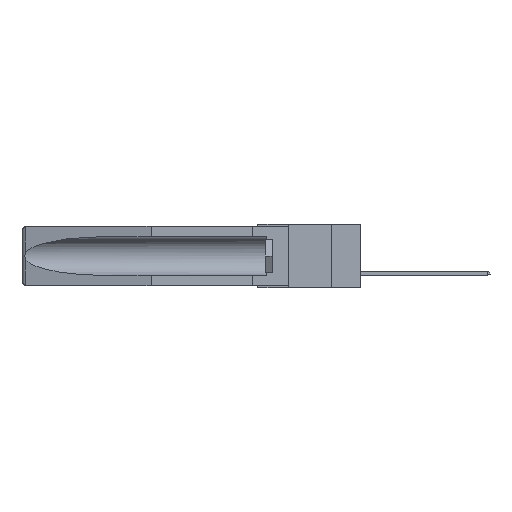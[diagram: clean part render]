
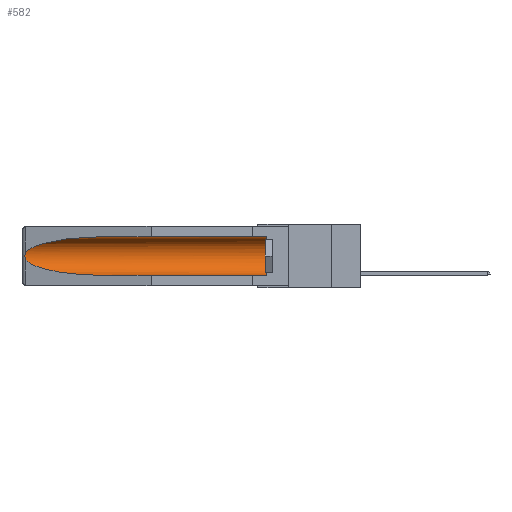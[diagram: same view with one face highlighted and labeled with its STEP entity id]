
A CAD part, left-side view. The second image highlights one B-rep face of the part: STEP entity #582.
In plain terms, the highlighted cylindrical face has radius 2.857 mm (diameter 5.715 mm), a partial arc.
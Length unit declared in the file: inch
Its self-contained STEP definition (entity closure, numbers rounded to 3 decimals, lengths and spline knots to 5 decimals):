
#582 = ADVANCED_FACE ( 'NONE', ( #4923 ), #21378, .F. ) ;
#949 = VECTOR ( 'NONE', #17998, 39.37008 ) ;
#1473 = DIRECTION ( 'NONE',  ( 0., -1., 0. ) ) ;
#1710 = VERTEX_POINT ( 'NONE', #6869 ) ;
#1951 = CARTESIAN_POINT ( 'NONE',  ( 0.155, -0.30754, -0.059 ) ) ;
#2475 = VERTEX_POINT ( 'NONE', #14850 ) ;
#3627 = EDGE_CURVE ( 'NONE', #15139, #6331, #18599, .T. ) ;
#3898 = ORIENTED_EDGE ( 'NONE', *, *, #20025, .T. ) ;
#4001 = CARTESIAN_POINT ( 'NONE',  ( 0.21114, 1.30732, -0.284 ) ) ;
#4146 = CARTESIAN_POINT ( 'NONE',  ( 0.26537, 1.52718, -0.19328 ) ) ;
#4448 = CARTESIAN_POINT ( 'NONE',  ( 0.155, 0.126, -0.1715 ) ) ;
#4598 = CARTESIAN_POINT ( 'NONE',  ( 0.21114, 1.30732, -0.059 ) ) ;
#4875 = CARTESIAN_POINT ( 'NONE',  ( 0.2675, 1.53308, -0.16763 ) ) ;
#4923 = FACE_OUTER_BOUND ( 'NONE', #17020, .T. ) ;
#5593 = CARTESIAN_POINT ( 'NONE',  ( 0.155, 0.126, -0.284 ) ) ;
#5659 = CARTESIAN_POINT ( 'NONE',  ( 0.155, 1.07973, -0.284 ) ) ;
#6331 = VERTEX_POINT ( 'NONE', #11270 ) ;
#6444 = CARTESIAN_POINT ( 'NONE',  ( 0.26537, 1.52718, -0.14972 ) ) ;
#6560 = CARTESIAN_POINT ( 'NONE',  ( 0.26537, 1.52718, -0.19328 ) ) ;
#6869 = CARTESIAN_POINT ( 'NONE',  ( 0.155, 1.07973, -0.059 ) ) ;
#7291 = DIRECTION ( 'NONE',  ( 0., 0., 1. ) ) ;
#7807 = LINE ( 'NONE', #10549, #949 ) ;
#8117 = ORIENTED_EDGE ( 'NONE', *, *, #3627, .T. ) ;
#8241 = CARTESIAN_POINT ( 'NONE',  ( 0.26597, 1.52961, -0.15275 ) ) ;
#8343 = VERTEX_POINT ( 'NONE', #21174 ) ;
#8438 = DIRECTION ( 'NONE',  ( 0., 0., 1. ) ) ;
#8598 = CIRCLE ( 'NONE', #20613, 0.1125 ) ;
#8803 = CARTESIAN_POINT ( 'NONE',  ( 0.155, -0.30754, -0.1715 ) ) ;
#10549 = CARTESIAN_POINT ( 'NONE',  ( 0.155, -0.30754, -0.284 ) ) ;
#11270 = CARTESIAN_POINT ( 'NONE',  ( 0.155, 1.07973, -0.284 ) ) ;
#11686 = CARTESIAN_POINT ( 'NONE',  ( 0.26654, 1.53092, -0.15636 ) ) ;
#11758 = CARTESIAN_POINT ( 'NONE',  ( 0.2675, 1.53308, -0.17534 ) ) ;
#11852 = ORIENTED_EDGE ( 'NONE', *, *, #21863, .T. ) ;
#11868 = CARTESIAN_POINT ( 'NONE',  ( 0.25451, 1.48313, -0.09465 ) ) ;
#12127 = EDGE_CURVE ( 'NONE', #20824, #8343, #8598, .T. ) ;
#12550 = B_SPLINE_CURVE_WITH_KNOTS ( 'NONE', 3,
 ( #18859, #8241, #11686, #17061, #4875, #11758, #22452, #15083, #17138, #6560 ),
 .UNSPECIFIED., .F., .F.,
 ( 4, 2, 2, 2, 4 ),
 ( 0., 0.00029, 0.00058, 0.00087, 0.00117 ),
 .UNSPECIFIED. ) ;
#12604 = VECTOR ( 'NONE', #16889, 39.37008 ) ;
#12777 = CARTESIAN_POINT ( 'NONE',  ( 0.25451, 1.48313, -0.24835 ) ) ;
#13032 = EDGE_CURVE ( 'NONE', #20824, #6331, #7807, .T. ) ;
#13405 = CARTESIAN_POINT ( 'NONE',  ( 0.155, 1.07973, -0.059 ) ) ;
#13868 = ORIENTED_EDGE ( 'NONE', *, *, #12127, .T. ) ;
#14570 = LINE ( 'NONE', #1951, #12604 ) ;
#14850 = CARTESIAN_POINT ( 'NONE',  ( 0.26537, 1.52718, -0.14972 ) ) ;
#14894 = ORIENTED_EDGE ( 'NONE', *, *, #15727, .T. ) ;
#15083 = CARTESIAN_POINT ( 'NONE',  ( 0.26655, 1.53094, -0.18657 ) ) ;
#15139 = VERTEX_POINT ( 'NONE', #16618 ) ;
#15166 = ORIENTED_EDGE ( 'NONE', *, *, #13032, .F. ) ;
#15727 = EDGE_CURVE ( 'NONE', #8343, #1710, #14570, .T. ) ;
#16618 = CARTESIAN_POINT ( 'NONE',  ( 0.26537, 1.52718, -0.19328 ) ) ;
#16889 = DIRECTION ( 'NONE',  ( 0., 1., 0. ) ) ;
#17020 = EDGE_LOOP ( 'NONE', ( #11852, #3898, #8117, #15166, #13868, #14894 ) ) ;
#17061 = CARTESIAN_POINT ( 'NONE',  ( 0.2673, 1.5327, -0.16383 ) ) ;
#17138 = CARTESIAN_POINT ( 'NONE',  ( 0.26597, 1.5296, -0.19026 ) ) ;
#17921 =( BOUNDED_CURVE ( )  B_SPLINE_CURVE ( 3, ( #13405, #4598, #11868, #6444 ),
 .UNSPECIFIED., .F., .F. ) 
 B_SPLINE_CURVE_WITH_KNOTS ( ( 4, 4 ),
 ( 4.71239, 6.08839 ),
 .UNSPECIFIED. ) 
 CURVE ( )  GEOMETRIC_REPRESENTATION_ITEM ( )  RATIONAL_B_SPLINE_CURVE ( ( 1., 0.848, 0.848, 1. ) ) 
 REPRESENTATION_ITEM ( '' )  );
#17998 = DIRECTION ( 'NONE',  ( 0., 1., 0. ) ) ;
#18599 =( BOUNDED_CURVE ( )  B_SPLINE_CURVE ( 3, ( #4146, #12777, #4001, #5659 ),
 .UNSPECIFIED., .F., .F. ) 
 B_SPLINE_CURVE_WITH_KNOTS ( ( 4, 4 ),
 ( 0.1948, 1.5708 ),
 .UNSPECIFIED. ) 
 CURVE ( )  GEOMETRIC_REPRESENTATION_ITEM ( )  RATIONAL_B_SPLINE_CURVE ( ( 1., 0.848, 0.848, 1. ) ) 
 REPRESENTATION_ITEM ( '' )  );
#18859 = CARTESIAN_POINT ( 'NONE',  ( 0.26537, 1.52718, -0.14972 ) ) ;
#19260 = AXIS2_PLACEMENT_3D ( 'NONE', #8803, #19373, #7291 ) ;
#19373 = DIRECTION ( 'NONE',  ( 0., 1., 0. ) ) ;
#20025 = EDGE_CURVE ( 'NONE', #2475, #15139, #12550, .T. ) ;
#20613 = AXIS2_PLACEMENT_3D ( 'NONE', #4448, #1473, #8438 ) ;
#20824 = VERTEX_POINT ( 'NONE', #5593 ) ;
#21174 = CARTESIAN_POINT ( 'NONE',  ( 0.155, 0.126, -0.059 ) ) ;
#21378 = CYLINDRICAL_SURFACE ( 'NONE', #19260, 0.1125 ) ;
#21863 = EDGE_CURVE ( 'NONE', #1710, #2475, #17921, .T. ) ;
#22452 = CARTESIAN_POINT ( 'NONE',  ( 0.2673, 1.53269, -0.17917 ) ) ;
